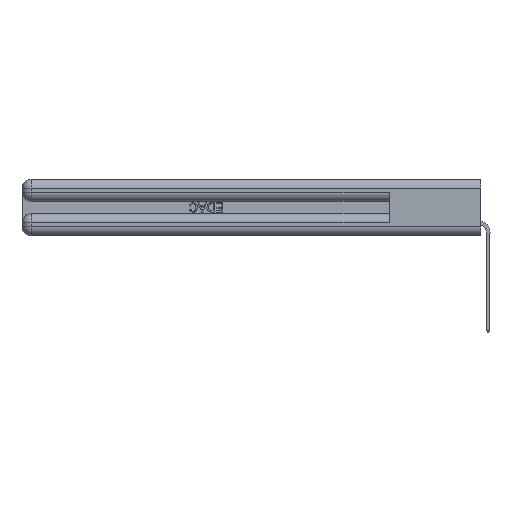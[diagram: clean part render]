
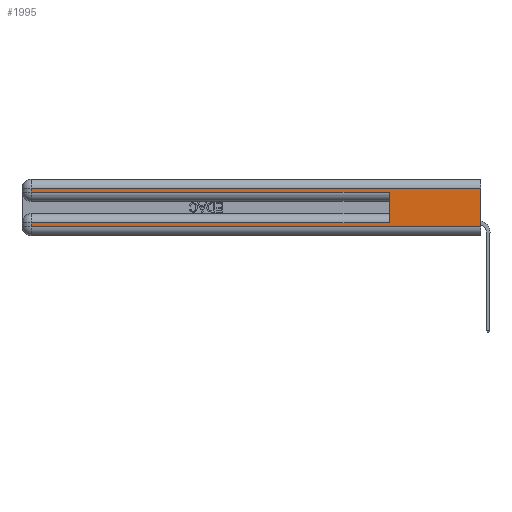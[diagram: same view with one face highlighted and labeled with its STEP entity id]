
A CAD part, left-side view. The second image highlights one B-rep face of the part: STEP entity #1995.
In plain terms, the highlighted planar face has unit normal (-1, 0, 0).
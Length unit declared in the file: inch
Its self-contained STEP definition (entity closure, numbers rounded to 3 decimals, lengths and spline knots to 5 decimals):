
#435 = LINE ( 'NONE', #39532, #39626 ) ;
#543 = VECTOR ( 'NONE', #26702, 39.37008 ) ;
#871 = ORIENTED_EDGE ( 'NONE', *, *, #27439, .T. ) ;
#996 = CARTESIAN_POINT ( 'NONE',  ( 0., 2.94, 0.06 ) ) ;
#1277 = PLANE ( 'NONE',  #4179 ) ;
#1698 = EDGE_CURVE ( 'NONE', #32810, #15773, #435, .T. ) ;
#1901 = CARTESIAN_POINT ( 'NONE',  ( 0., 0., 0.06 ) ) ;
#1924 = VECTOR ( 'NONE', #8052, 39.37008 ) ;
#1995 = ADVANCED_FACE ( 'NONE', ( #27974 ), #1277, .F. ) ;
#2397 = ORIENTED_EDGE ( 'NONE', *, *, #16611, .T. ) ;
#3678 = ORIENTED_EDGE ( 'NONE', *, *, #1698, .F. ) ;
#3725 = LINE ( 'NONE', #1901, #35686 ) ;
#4179 = AXIS2_PLACEMENT_3D ( 'NONE', #25445, #16521, #25579 ) ;
#4735 = VERTEX_POINT ( 'NONE', #38917 ) ;
#5862 = EDGE_CURVE ( 'NONE', #6743, #25704, #13411, .T. ) ;
#6743 = VERTEX_POINT ( 'NONE', #20774 ) ;
#8052 = DIRECTION ( 'NONE',  ( 0., 1., 0. ) ) ;
#8661 = CARTESIAN_POINT ( 'NONE',  ( 0., 2.94, 0.37 ) ) ;
#9471 = LINE ( 'NONE', #12652, #31210 ) ;
#9899 = VECTOR ( 'NONE', #28792, 39.37008 ) ;
#10378 = VECTOR ( 'NONE', #16425, 39.37008 ) ;
#10722 = EDGE_CURVE ( 'NONE', #32810, #23101, #34137, .T. ) ;
#12652 = CARTESIAN_POINT ( 'NONE',  ( 0., 2.94, 0.37 ) ) ;
#13411 = LINE ( 'NONE', #8661, #21279 ) ;
#14257 = DIRECTION ( 'NONE',  ( 0., -1., 0. ) ) ;
#14294 = LINE ( 'NONE', #19536, #9899 ) ;
#15248 = ORIENTED_EDGE ( 'NONE', *, *, #37158, .T. ) ;
#15651 = VERTEX_POINT ( 'NONE', #16822 ) ;
#15773 = VERTEX_POINT ( 'NONE', #34745 ) ;
#16301 = VERTEX_POINT ( 'NONE', #996 ) ;
#16425 = DIRECTION ( 'NONE',  ( 0., 1., 0. ) ) ;
#16521 = DIRECTION ( 'NONE',  ( 1., 0., 0. ) ) ;
#16611 = EDGE_CURVE ( 'NONE', #25704, #15773, #14294, .T. ) ;
#16822 = CARTESIAN_POINT ( 'NONE',  ( 0., 0., 0.31 ) ) ;
#17783 = ORIENTED_EDGE ( 'NONE', *, *, #5862, .T. ) ;
#18797 = LINE ( 'NONE', #39223, #1924 ) ;
#19536 = CARTESIAN_POINT ( 'NONE',  ( 0., 0., 0.285 ) ) ;
#20774 = CARTESIAN_POINT ( 'NONE',  ( 0., 2.94, 0.31 ) ) ;
#21120 = ORIENTED_EDGE ( 'NONE', *, *, #10722, .T. ) ;
#21279 = VECTOR ( 'NONE', #23816, 39.37008 ) ;
#21949 = EDGE_LOOP ( 'NONE', ( #27781, #35168, #17783, #2397, #3678, #21120, #15248, #871 ) ) ;
#23101 = VERTEX_POINT ( 'NONE', #31815 ) ;
#23816 = DIRECTION ( 'NONE',  ( 0., 0., -1. ) ) ;
#24906 = DIRECTION ( 'NONE',  ( 0., 0., -1. ) ) ;
#25000 = EDGE_CURVE ( 'NONE', #15651, #4735, #25734, .T. ) ;
#25445 = CARTESIAN_POINT ( 'NONE',  ( 0., 0., 0.37 ) ) ;
#25579 = DIRECTION ( 'NONE',  ( 0., 0., -1. ) ) ;
#25616 = CARTESIAN_POINT ( 'NONE',  ( 0., 0., 0.085 ) ) ;
#25704 = VERTEX_POINT ( 'NONE', #35845 ) ;
#25734 = LINE ( 'NONE', #36037, #543 ) ;
#26702 = DIRECTION ( 'NONE',  ( 0., 0., -1. ) ) ;
#27439 = EDGE_CURVE ( 'NONE', #16301, #4735, #3725, .T. ) ;
#27513 = DIRECTION ( 'NONE',  ( 0., 0., 1. ) ) ;
#27781 = ORIENTED_EDGE ( 'NONE', *, *, #25000, .F. ) ;
#27974 = FACE_OUTER_BOUND ( 'NONE', #21949, .T. ) ;
#28792 = DIRECTION ( 'NONE',  ( 0., -1., 0. ) ) ;
#31210 = VECTOR ( 'NONE', #24906, 39.37008 ) ;
#31815 = CARTESIAN_POINT ( 'NONE',  ( 0., 2.94, 0.085 ) ) ;
#32810 = VERTEX_POINT ( 'NONE', #39568 ) ;
#34137 = LINE ( 'NONE', #25616, #10378 ) ;
#34317 = EDGE_CURVE ( 'NONE', #15651, #6743, #18797, .T. ) ;
#34745 = CARTESIAN_POINT ( 'NONE',  ( 0., 0.6, 0.285 ) ) ;
#35168 = ORIENTED_EDGE ( 'NONE', *, *, #34317, .T. ) ;
#35686 = VECTOR ( 'NONE', #14257, 39.37008 ) ;
#35845 = CARTESIAN_POINT ( 'NONE',  ( 0., 2.94, 0.285 ) ) ;
#36037 = CARTESIAN_POINT ( 'NONE',  ( 0., 0., 0.37 ) ) ;
#37158 = EDGE_CURVE ( 'NONE', #23101, #16301, #9471, .T. ) ;
#38917 = CARTESIAN_POINT ( 'NONE',  ( 0., 0., 0.06 ) ) ;
#39223 = CARTESIAN_POINT ( 'NONE',  ( 0., 0., 0.31 ) ) ;
#39532 = CARTESIAN_POINT ( 'NONE',  ( 0., 0.6, 0.145 ) ) ;
#39568 = CARTESIAN_POINT ( 'NONE',  ( 0., 0.6, 0.085 ) ) ;
#39626 = VECTOR ( 'NONE', #27513, 39.37008 ) ;
